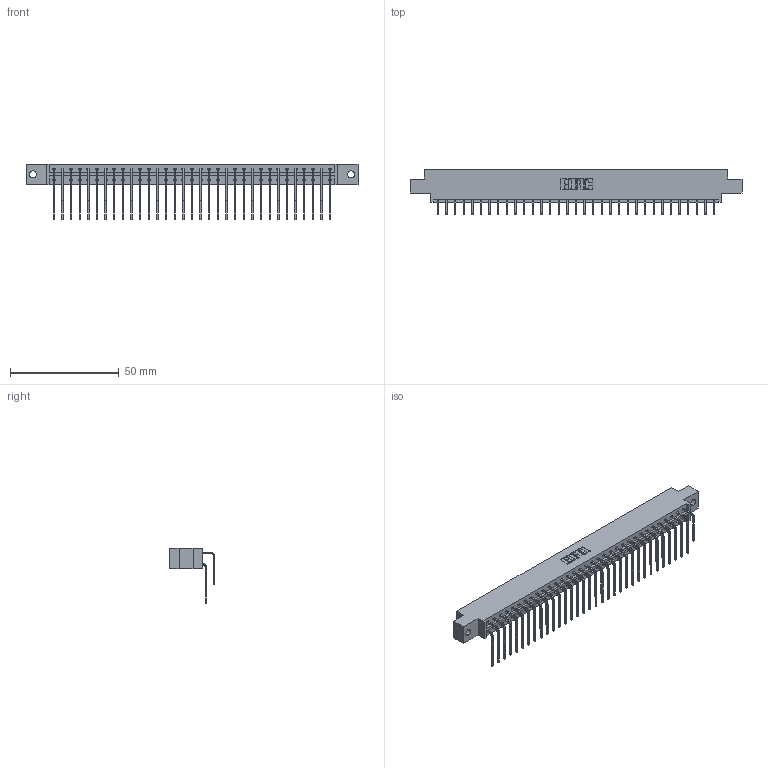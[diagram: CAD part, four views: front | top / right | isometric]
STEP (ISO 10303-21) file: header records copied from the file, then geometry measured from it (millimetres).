
FILE_DESCRIPTION (( 'STEP AP203' ), '1' );
FILE_NAME ('833-066-559-802.STEP', '2020-06-05T09:44:26', ( '' ), ( '' ), 'SwSTEP 2.0', 'SolidWorks 2020', '' );
FILE_SCHEMA (( 'CONFIG_CONTROL_DESIGN' ));
Length unit declared in the file: inch
Products named in the file (4): 345-292-001_558 559 Tail - 1; 345-292-001_559 Tail - 2; 833 Part_Offset - .128 Dia; 833-066-559-802
Assembly tree (67 placements, depth 2):
  833-066-559-802
    833 Part_Offset - .128 Dia
    345-292-001_558 559 Tail - 1  x33
    345-292-001_559 Tail - 2  x33
Bounding box: 152.3 x 20.9 x 25.53 mm (x, y, z)
Volume: 15580.9 mm3; surface area: 20167.7 mm2
Topology: 67 solids, 67 shells, 3682 faces, 10949 edges, 7210 vertices
Faces by surface type: plane 2582, cylinder 1100
Entity records: 24313 total; most frequent: CARTESIAN_POINT 4093, ORIENTED_EDGE 3978, DIRECTION 3493, EDGE_CURVE 1989, LINE 1821, VECTOR 1821, VERTEX_POINT 1322, AXIS2_PLACEMENT_3D 836
